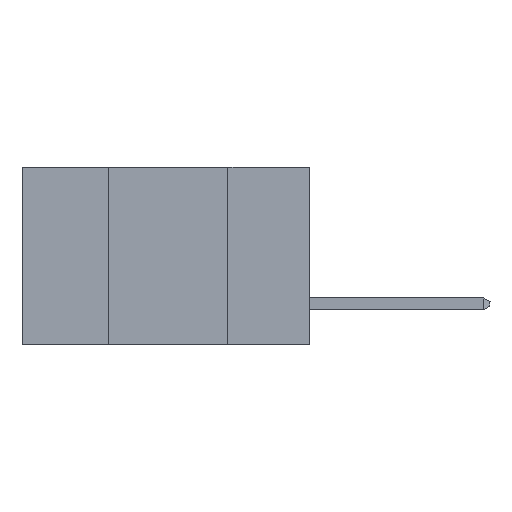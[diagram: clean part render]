
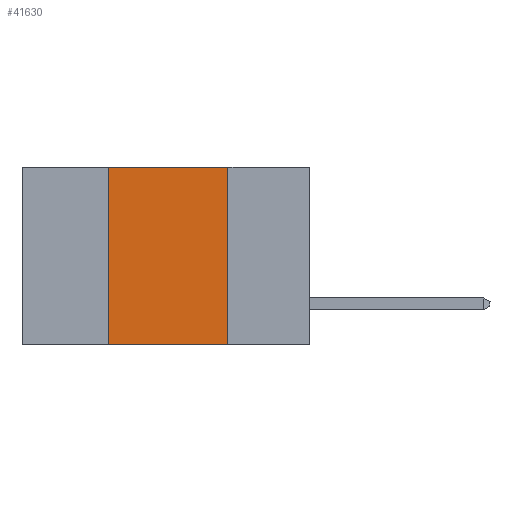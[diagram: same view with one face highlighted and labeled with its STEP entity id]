
A CAD part, left-side view. The second image highlights one B-rep face of the part: STEP entity #41630.
In plain terms, the highlighted planar face has unit normal (-1, 0, 0).
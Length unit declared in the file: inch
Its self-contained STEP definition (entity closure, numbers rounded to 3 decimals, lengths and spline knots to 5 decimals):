
#2020 = DIRECTION ( 'NONE',  ( 0., 0., 1. ) ) ;
#2479 = LINE ( 'NONE', #31714, #43491 ) ;
#4670 = ORIENTED_EDGE ( 'NONE', *, *, #4891, .F. ) ;
#4891 = EDGE_CURVE ( 'NONE', #6585, #20337, #39067, .T. ) ;
#6585 = VERTEX_POINT ( 'NONE', #9494 ) ;
#6843 = LINE ( 'NONE', #29874, #46204 ) ;
#7072 = EDGE_CURVE ( 'NONE', #43154, #14769, #6843, .T. ) ;
#9494 = CARTESIAN_POINT ( 'NONE',  ( 0., 0.42, -0.37 ) ) ;
#11755 = CARTESIAN_POINT ( 'NONE',  ( 0., 0.6, -0.37 ) ) ;
#13788 = EDGE_CURVE ( 'NONE', #20337, #43154, #2479, .T. ) ;
#14689 = EDGE_CURVE ( 'NONE', #6585, #14769, #31673, .T. ) ;
#14769 = VERTEX_POINT ( 'NONE', #24098 ) ;
#15638 = EDGE_LOOP ( 'NONE', ( #20554, #30048, #4670, #38053 ) ) ;
#17406 = DIRECTION ( 'NONE',  ( 0., -1., 0. ) ) ;
#17761 = DIRECTION ( 'NONE',  ( 0., -1., 0. ) ) ;
#20337 = VERTEX_POINT ( 'NONE', #36600 ) ;
#20554 = ORIENTED_EDGE ( 'NONE', *, *, #7072, .F. ) ;
#24098 = CARTESIAN_POINT ( 'NONE',  ( 0., 0.17, -0.37 ) ) ;
#25029 = VECTOR ( 'NONE', #2020, 39.37008 ) ;
#25516 = CARTESIAN_POINT ( 'NONE',  ( 0., 0.17, 0. ) ) ;
#27637 = CARTESIAN_POINT ( 'NONE',  ( 0., 0.42, 0. ) ) ;
#28265 = VECTOR ( 'NONE', #17761, 39.37008 ) ;
#28702 = DIRECTION ( 'NONE',  ( 1., 0., 0. ) ) ;
#29874 = CARTESIAN_POINT ( 'NONE',  ( 0., 0.17, 0. ) ) ;
#30048 = ORIENTED_EDGE ( 'NONE', *, *, #13788, .F. ) ;
#30807 = FACE_OUTER_BOUND ( 'NONE', #15638, .T. ) ;
#31673 = LINE ( 'NONE', #11755, #28265 ) ;
#31714 = CARTESIAN_POINT ( 'NONE',  ( 0., 0.6, 0. ) ) ;
#31840 = CARTESIAN_POINT ( 'NONE',  ( 0., 0.6, 0. ) ) ;
#36600 = CARTESIAN_POINT ( 'NONE',  ( 0., 0.42, 0. ) ) ;
#37099 = DIRECTION ( 'NONE',  ( 0., 0., -1. ) ) ;
#38053 = ORIENTED_EDGE ( 'NONE', *, *, #14689, .T. ) ;
#38112 = AXIS2_PLACEMENT_3D ( 'NONE', #31840, #28702, #39374 ) ;
#39067 = LINE ( 'NONE', #27637, #25029 ) ;
#39374 = DIRECTION ( 'NONE',  ( 0., 0., -1. ) ) ;
#41630 = ADVANCED_FACE ( 'NONE', ( #30807 ), #42997, .F. ) ;
#42997 = PLANE ( 'NONE',  #38112 ) ;
#43154 = VERTEX_POINT ( 'NONE', #25516 ) ;
#43491 = VECTOR ( 'NONE', #17406, 39.37008 ) ;
#46204 = VECTOR ( 'NONE', #37099, 39.37008 ) ;
